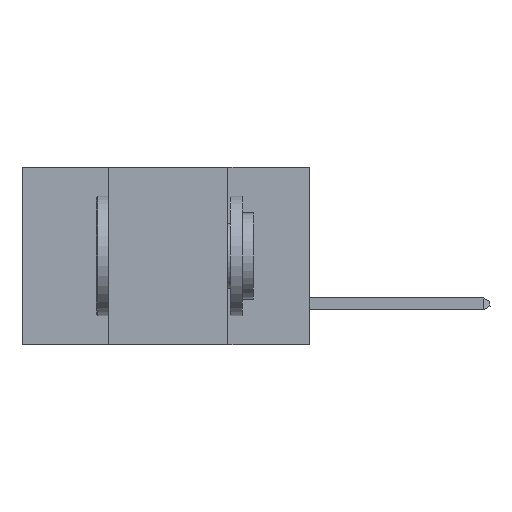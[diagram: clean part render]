
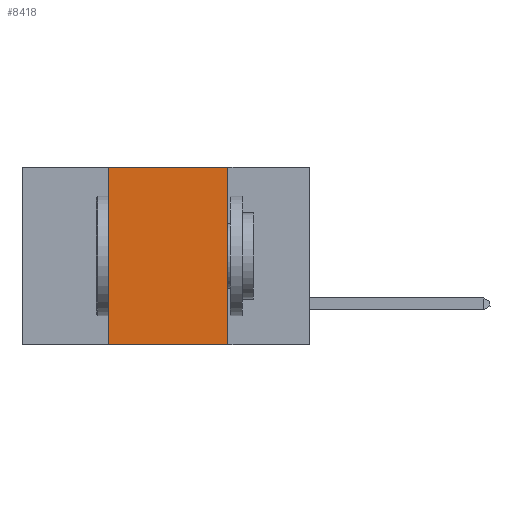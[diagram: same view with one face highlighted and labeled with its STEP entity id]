
A CAD part, left-side view. The second image highlights one B-rep face of the part: STEP entity #8418.
In plain terms, the highlighted planar face has unit normal (-1, 0, 0).
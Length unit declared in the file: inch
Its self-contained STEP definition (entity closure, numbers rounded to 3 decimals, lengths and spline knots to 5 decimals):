
#443 = EDGE_CURVE ( 'NONE', #7269, #10374, #4141, .T. ) ;
#912 = FACE_OUTER_BOUND ( 'NONE', #6064, .T. ) ;
#1342 = ORIENTED_EDGE ( 'NONE', *, *, #7829, .F. ) ;
#1497 = EDGE_CURVE ( 'NONE', #2294, #7269, #4256, .T. ) ;
#1855 = CARTESIAN_POINT ( 'NONE',  ( 0., 0.42, 0. ) ) ;
#1859 = VECTOR ( 'NONE', #10168, 39.37008 ) ;
#2018 = EDGE_CURVE ( 'NONE', #12321, #10374, #5716, .T. ) ;
#2101 = DIRECTION ( 'NONE',  ( 0., 0., 1. ) ) ;
#2294 = VERTEX_POINT ( 'NONE', #1855 ) ;
#2518 = VECTOR ( 'NONE', #8690, 39.37008 ) ;
#3374 = CARTESIAN_POINT ( 'NONE',  ( 0., 0.6, -0.37 ) ) ;
#3783 = PLANE ( 'NONE',  #6334 ) ;
#4141 = LINE ( 'NONE', #5641, #2518 ) ;
#4256 = LINE ( 'NONE', #9150, #1859 ) ;
#4908 = DIRECTION ( 'NONE',  ( 1., 0., 0. ) ) ;
#5546 = VECTOR ( 'NONE', #12613, 39.37008 ) ;
#5641 = CARTESIAN_POINT ( 'NONE',  ( 0., 0.17, 0. ) ) ;
#5716 = LINE ( 'NONE', #3374, #5546 ) ;
#5797 = ORIENTED_EDGE ( 'NONE', *, *, #443, .F. ) ;
#6064 = EDGE_LOOP ( 'NONE', ( #5797, #8353, #1342, #12329 ) ) ;
#6334 = AXIS2_PLACEMENT_3D ( 'NONE', #11912, #4908, #6853 ) ;
#6853 = DIRECTION ( 'NONE',  ( 0., 0., -1. ) ) ;
#7063 = CARTESIAN_POINT ( 'NONE',  ( 0., 0.17, -0.37 ) ) ;
#7269 = VERTEX_POINT ( 'NONE', #13209 ) ;
#7829 = EDGE_CURVE ( 'NONE', #12321, #2294, #12159, .T. ) ;
#8353 = ORIENTED_EDGE ( 'NONE', *, *, #1497, .F. ) ;
#8418 = ADVANCED_FACE ( 'NONE', ( #912 ), #3783, .F. ) ;
#8690 = DIRECTION ( 'NONE',  ( 0., 0., -1. ) ) ;
#9150 = CARTESIAN_POINT ( 'NONE',  ( 0., 0.6, 0. ) ) ;
#10168 = DIRECTION ( 'NONE',  ( 0., -1., 0. ) ) ;
#10374 = VERTEX_POINT ( 'NONE', #7063 ) ;
#10679 = CARTESIAN_POINT ( 'NONE',  ( 0., 0.42, -0.37 ) ) ;
#11912 = CARTESIAN_POINT ( 'NONE',  ( 0., 0.6, 0. ) ) ;
#12159 = LINE ( 'NONE', #12330, #12944 ) ;
#12321 = VERTEX_POINT ( 'NONE', #10679 ) ;
#12329 = ORIENTED_EDGE ( 'NONE', *, *, #2018, .T. ) ;
#12330 = CARTESIAN_POINT ( 'NONE',  ( 0., 0.42, 0. ) ) ;
#12613 = DIRECTION ( 'NONE',  ( 0., -1., 0. ) ) ;
#12944 = VECTOR ( 'NONE', #2101, 39.37008 ) ;
#13209 = CARTESIAN_POINT ( 'NONE',  ( 0., 0.17, 0. ) ) ;
